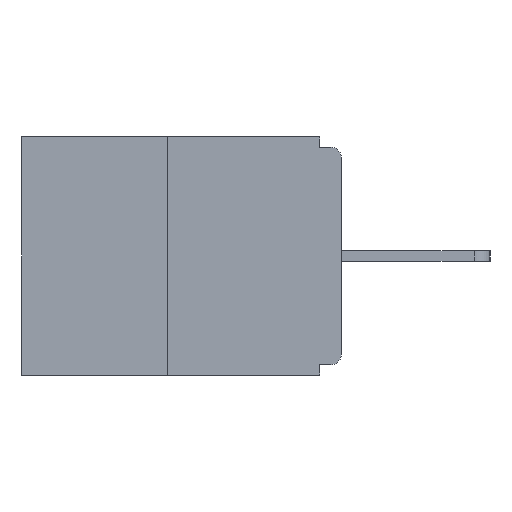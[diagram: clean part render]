
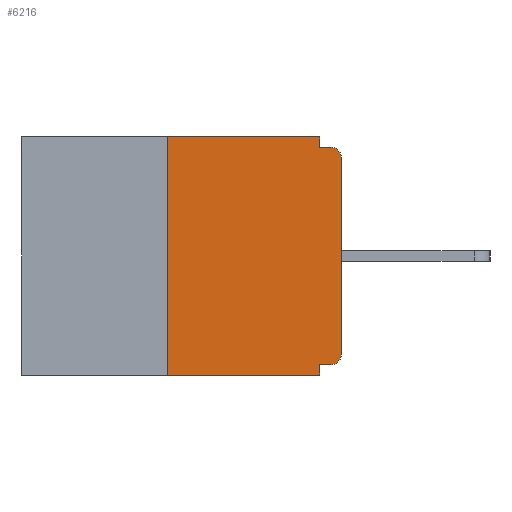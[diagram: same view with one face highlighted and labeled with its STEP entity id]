
A CAD part, left-side view. The second image highlights one B-rep face of the part: STEP entity #6216.
In plain terms, the highlighted planar face has unit normal (-1, 0, 0).
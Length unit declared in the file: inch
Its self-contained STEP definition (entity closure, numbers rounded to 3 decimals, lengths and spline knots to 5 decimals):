
#202 = ORIENTED_EDGE ( 'NONE', *, *, #2490, .T. ) ;
#509 = DIRECTION ( 'NONE',  ( -1., 0., 0. ) ) ;
#961 = CARTESIAN_POINT ( 'NONE',  ( 0., 0.031, 0. ) ) ;
#976 = EDGE_CURVE ( 'NONE', #14961, #10427, #18009, .T. ) ;
#983 = DIRECTION ( 'NONE',  ( 0., 0., 1. ) ) ;
#1037 = VECTOR ( 'NONE', #10915, 39.37008 ) ;
#1110 = DIRECTION ( 'NONE',  ( 0., 0., -1. ) ) ;
#1431 = DIRECTION ( 'NONE',  ( 0., 1., 0. ) ) ;
#1865 = DIRECTION ( 'NONE',  ( 0., -1., 0. ) ) ;
#2490 = EDGE_CURVE ( 'NONE', #5925, #20821, #20622, .T. ) ;
#2566 = CARTESIAN_POINT ( 'NONE',  ( 0., 0., -0.03 ) ) ;
#2849 = AXIS2_PLACEMENT_3D ( 'NONE', #24054, #14650, #16877 ) ;
#2924 = DIRECTION ( 'NONE',  ( -1., 0., 0. ) ) ;
#3007 = LINE ( 'NONE', #17019, #7993 ) ;
#3029 = VECTOR ( 'NONE', #8368, 39.37008 ) ;
#3119 = EDGE_CURVE ( 'NONE', #14961, #19844, #21166, .T. ) ;
#3314 = CIRCLE ( 'NONE', #8954, 0.015 ) ;
#3702 = PLANE ( 'NONE',  #2849 ) ;
#4100 = ORIENTED_EDGE ( 'NONE', *, *, #7112, .T. ) ;
#4275 = LINE ( 'NONE', #14598, #19443 ) ;
#4514 = CARTESIAN_POINT ( 'NONE',  ( 0., 0., -0.313 ) ) ;
#5356 = LINE ( 'NONE', #961, #5919 ) ;
#5919 = VECTOR ( 'NONE', #17818, 39.37008 ) ;
#5925 = VERTEX_POINT ( 'NONE', #14065 ) ;
#6167 = EDGE_LOOP ( 'NONE', ( #15678, #21984, #19231, #11562, #17091, #202, #21100, #4100, #9295, #17285 ) ) ;
#6216 = ADVANCED_FACE ( 'NONE', ( #8602 ), #3702, .F. ) ;
#7084 = DIRECTION ( 'NONE',  ( 0., 0., -1. ) ) ;
#7112 = EDGE_CURVE ( 'NONE', #7431, #22354, #3314, .T. ) ;
#7259 = CARTESIAN_POINT ( 'NONE',  ( 0., 0.031, 0. ) ) ;
#7431 = VERTEX_POINT ( 'NONE', #2566 ) ;
#7993 = VECTOR ( 'NONE', #1865, 39.37008 ) ;
#8139 = CARTESIAN_POINT ( 'NONE',  ( 0., 0.031, -0.343 ) ) ;
#8368 = DIRECTION ( 'NONE',  ( 0., 0., 1. ) ) ;
#8602 = FACE_OUTER_BOUND ( 'NONE', #6167, .T. ) ;
#8954 = AXIS2_PLACEMENT_3D ( 'NONE', #12209, #2924, #1110 ) ;
#9295 = ORIENTED_EDGE ( 'NONE', *, *, #11502, .F. ) ;
#9305 = EDGE_CURVE ( 'NONE', #19844, #17364, #3007, .T. ) ;
#10103 = CARTESIAN_POINT ( 'NONE',  ( 0., 0.25, -0.343 ) ) ;
#10427 = VERTEX_POINT ( 'NONE', #8139 ) ;
#10566 = DIRECTION ( 'NONE',  ( 0., -1., 0. ) ) ;
#10799 = CARTESIAN_POINT ( 'NONE',  ( 0., 0.031, -0.343 ) ) ;
#10915 = DIRECTION ( 'NONE',  ( 0., -1., 0. ) ) ;
#11317 = VECTOR ( 'NONE', #7084, 39.37008 ) ;
#11347 = VERTEX_POINT ( 'NONE', #17474 ) ;
#11358 = CARTESIAN_POINT ( 'NONE',  ( 0., 0.031, -0.328 ) ) ;
#11502 = EDGE_CURVE ( 'NONE', #11347, #22354, #4275, .T. ) ;
#11562 = ORIENTED_EDGE ( 'NONE', *, *, #23578, .F. ) ;
#12017 = DIRECTION ( 'NONE',  ( 0., 0., -1. ) ) ;
#12030 = VECTOR ( 'NONE', #983, 39.37008 ) ;
#12209 = CARTESIAN_POINT ( 'NONE',  ( 0., 0.015, -0.03 ) ) ;
#13581 = EDGE_CURVE ( 'NONE', #17364, #11347, #5356, .T. ) ;
#14065 = CARTESIAN_POINT ( 'NONE',  ( 0., 0.015, -0.328 ) ) ;
#14598 = CARTESIAN_POINT ( 'NONE',  ( 0., 0., -0.015 ) ) ;
#14650 = DIRECTION ( 'NONE',  ( 1., 0., 0. ) ) ;
#14961 = VERTEX_POINT ( 'NONE', #10103 ) ;
#15476 = CARTESIAN_POINT ( 'NONE',  ( 0., 0.25, 0. ) ) ;
#15479 = CARTESIAN_POINT ( 'NONE',  ( 0., 0.015, -0.313 ) ) ;
#15678 = ORIENTED_EDGE ( 'NONE', *, *, #9305, .F. ) ;
#16877 = DIRECTION ( 'NONE',  ( 0., 0., -1. ) ) ;
#17019 = CARTESIAN_POINT ( 'NONE',  ( 0., 0.46, 0. ) ) ;
#17054 = LINE ( 'NONE', #19796, #12030 ) ;
#17091 = ORIENTED_EDGE ( 'NONE', *, *, #17427, .F. ) ;
#17123 = AXIS2_PLACEMENT_3D ( 'NONE', #15479, #509, #12017 ) ;
#17285 = ORIENTED_EDGE ( 'NONE', *, *, #13581, .F. ) ;
#17315 = VECTOR ( 'NONE', #1431, 39.37008 ) ;
#17364 = VERTEX_POINT ( 'NONE', #7259 ) ;
#17427 = EDGE_CURVE ( 'NONE', #5925, #22766, #24035, .T. ) ;
#17474 = CARTESIAN_POINT ( 'NONE',  ( 0., 0.031, -0.015 ) ) ;
#17818 = DIRECTION ( 'NONE',  ( 0., 0., -1. ) ) ;
#18009 = LINE ( 'NONE', #22125, #1037 ) ;
#18076 = LINE ( 'NONE', #10799, #11317 ) ;
#18392 = CARTESIAN_POINT ( 'NONE',  ( 0., 0.25, 0. ) ) ;
#19231 = ORIENTED_EDGE ( 'NONE', *, *, #976, .T. ) ;
#19443 = VECTOR ( 'NONE', #10566, 39.37008 ) ;
#19796 = CARTESIAN_POINT ( 'NONE',  ( 0., 0., 0. ) ) ;
#19844 = VERTEX_POINT ( 'NONE', #18392 ) ;
#20321 = CARTESIAN_POINT ( 'NONE',  ( 0., 0., -0.328 ) ) ;
#20479 = EDGE_CURVE ( 'NONE', #20821, #7431, #17054, .T. ) ;
#20622 = CIRCLE ( 'NONE', #17123, 0.015 ) ;
#20821 = VERTEX_POINT ( 'NONE', #4514 ) ;
#21100 = ORIENTED_EDGE ( 'NONE', *, *, #20479, .T. ) ;
#21166 = LINE ( 'NONE', #15476, #3029 ) ;
#21984 = ORIENTED_EDGE ( 'NONE', *, *, #3119, .F. ) ;
#22125 = CARTESIAN_POINT ( 'NONE',  ( 0., 0.46, -0.343 ) ) ;
#22354 = VERTEX_POINT ( 'NONE', #22584 ) ;
#22584 = CARTESIAN_POINT ( 'NONE',  ( 0., 0.015, -0.015 ) ) ;
#22766 = VERTEX_POINT ( 'NONE', #11358 ) ;
#23578 = EDGE_CURVE ( 'NONE', #22766, #10427, #18076, .T. ) ;
#24035 = LINE ( 'NONE', #20321, #17315 ) ;
#24054 = CARTESIAN_POINT ( 'NONE',  ( 0., 0.46, 0. ) ) ;
